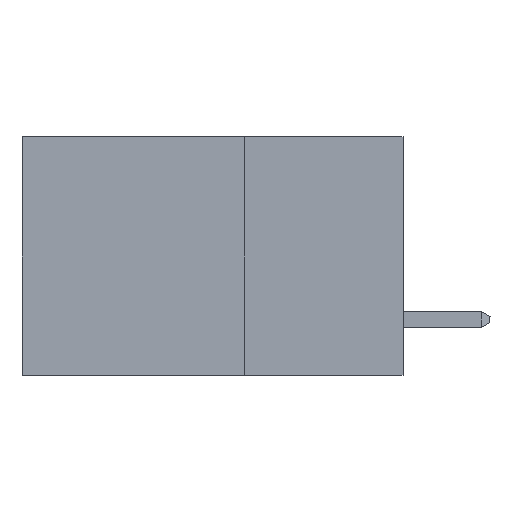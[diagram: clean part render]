
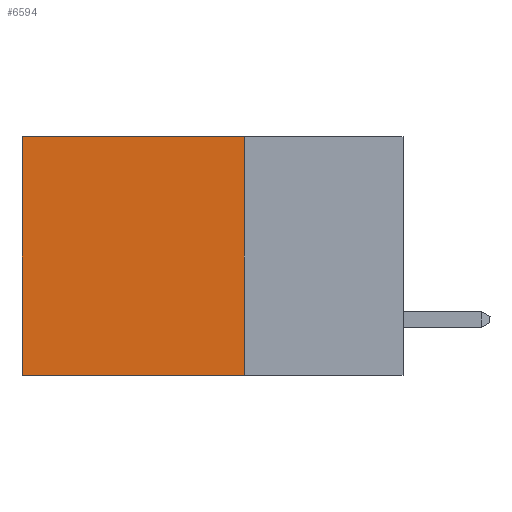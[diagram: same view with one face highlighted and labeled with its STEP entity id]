
A CAD part, left-side view. The second image highlights one B-rep face of the part: STEP entity #6594.
In plain terms, the highlighted planar face has unit normal (-1, 0, 0).
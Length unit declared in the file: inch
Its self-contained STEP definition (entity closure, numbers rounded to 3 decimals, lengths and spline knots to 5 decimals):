
#358 = VERTEX_POINT ( 'NONE', #6115 ) ;
#546 = CARTESIAN_POINT ( 'NONE',  ( 0.2875, 0.25, -0.375 ) ) ;
#724 = DIRECTION ( 'NONE',  ( 0., 1., 0. ) ) ;
#771 = CARTESIAN_POINT ( 'NONE',  ( 0.2875, 0.25, 0. ) ) ;
#831 = EDGE_CURVE ( 'NONE', #2917, #358, #2133, .T. ) ;
#855 = DIRECTION ( 'NONE',  ( 0., 0., -1. ) ) ;
#857 = VECTOR ( 'NONE', #724, 39.37008 ) ;
#1255 = ORIENTED_EDGE ( 'NONE', *, *, #6722, .T. ) ;
#1664 = AXIS2_PLACEMENT_3D ( 'NONE', #3503, #4712, #855 ) ;
#1894 = CARTESIAN_POINT ( 'NONE',  ( 0.2875, 0.6, -0.375 ) ) ;
#2133 = LINE ( 'NONE', #546, #4056 ) ;
#2323 = FACE_OUTER_BOUND ( 'NONE', #5662, .T. ) ;
#2415 = VECTOR ( 'NONE', #7836, 39.37008 ) ;
#2596 = EDGE_CURVE ( 'NONE', #358, #7464, #5941, .T. ) ;
#2917 = VERTEX_POINT ( 'NONE', #8324 ) ;
#3044 = CARTESIAN_POINT ( 'NONE',  ( 0.2875, 0.6, 0. ) ) ;
#3140 = DIRECTION ( 'NONE',  ( 0., 0., -1. ) ) ;
#3295 = DIRECTION ( 'NONE',  ( 0., 1., 0. ) ) ;
#3503 = CARTESIAN_POINT ( 'NONE',  ( 0.2875, 0.25, -0.375 ) ) ;
#4056 = VECTOR ( 'NONE', #3140, 39.37008 ) ;
#4686 = CARTESIAN_POINT ( 'NONE',  ( 0.2875, 0.6, -0.375 ) ) ;
#4712 = DIRECTION ( 'NONE',  ( 1., 0., 0. ) ) ;
#4739 = PLANE ( 'NONE',  #1664 ) ;
#5052 = VERTEX_POINT ( 'NONE', #3044 ) ;
#5196 = EDGE_CURVE ( 'NONE', #2917, #5052, #7219, .T. ) ;
#5282 = ORIENTED_EDGE ( 'NONE', *, *, #5196, .T. ) ;
#5662 = EDGE_LOOP ( 'NONE', ( #1255, #6660, #8187, #5282 ) ) ;
#5751 = VECTOR ( 'NONE', #3295, 39.37008 ) ;
#5941 = LINE ( 'NONE', #7152, #5751 ) ;
#6115 = CARTESIAN_POINT ( 'NONE',  ( 0.2875, 0.25, -0.375 ) ) ;
#6594 = ADVANCED_FACE ( 'NONE', ( #2323 ), #4739, .F. ) ;
#6660 = ORIENTED_EDGE ( 'NONE', *, *, #2596, .F. ) ;
#6722 = EDGE_CURVE ( 'NONE', #5052, #7464, #7800, .T. ) ;
#7152 = CARTESIAN_POINT ( 'NONE',  ( 0.2875, 0.25, -0.375 ) ) ;
#7219 = LINE ( 'NONE', #771, #857 ) ;
#7464 = VERTEX_POINT ( 'NONE', #1894 ) ;
#7800 = LINE ( 'NONE', #4686, #2415 ) ;
#7836 = DIRECTION ( 'NONE',  ( 0., 0., -1. ) ) ;
#8187 = ORIENTED_EDGE ( 'NONE', *, *, #831, .F. ) ;
#8324 = CARTESIAN_POINT ( 'NONE',  ( 0.2875, 0.25, 0. ) ) ;
